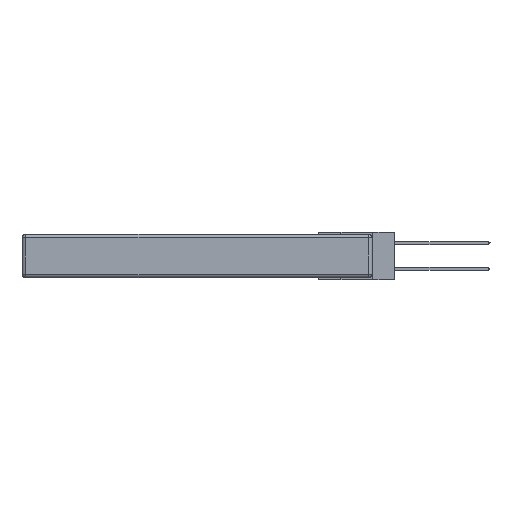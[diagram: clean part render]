
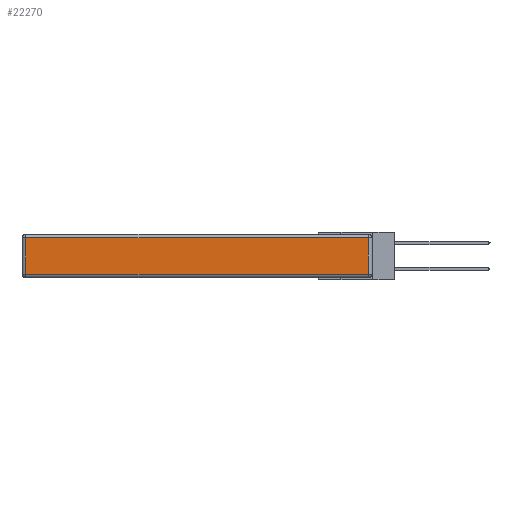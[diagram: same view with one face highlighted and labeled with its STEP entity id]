
A CAD part, left-side view. The second image highlights one B-rep face of the part: STEP entity #22270.
In plain terms, the highlighted planar face has unit normal (-1, 0, 0).
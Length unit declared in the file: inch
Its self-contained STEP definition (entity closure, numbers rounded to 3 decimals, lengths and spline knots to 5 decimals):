
#1316 = VERTEX_POINT ( 'NONE', #15758 ) ;
#3659 = CARTESIAN_POINT ( 'NONE',  ( 0., 2.72, -0.343 ) ) ;
#4221 = ORIENTED_EDGE ( 'NONE', *, *, #12453, .T. ) ;
#4222 = LINE ( 'NONE', #9980, #21115 ) ;
#4684 = CARTESIAN_POINT ( 'NONE',  ( 0., 0.03, -0.03 ) ) ;
#5134 = ORIENTED_EDGE ( 'NONE', *, *, #9528, .T. ) ;
#6177 = AXIS2_PLACEMENT_3D ( 'NONE', #9435, #19359, #13591 ) ;
#8628 = CARTESIAN_POINT ( 'NONE',  ( 0., 2.72, -0.03 ) ) ;
#9435 = CARTESIAN_POINT ( 'NONE',  ( 0., 0., -0.343 ) ) ;
#9528 = EDGE_CURVE ( 'NONE', #24288, #19897, #4222, .T. ) ;
#9539 = EDGE_CURVE ( 'NONE', #19897, #18191, #11582, .T. ) ;
#9980 = CARTESIAN_POINT ( 'NONE',  ( 0., 2.75, -0.03 ) ) ;
#10282 = VECTOR ( 'NONE', #20250, 39.37008 ) ;
#10869 = DIRECTION ( 'NONE',  ( 0., -1., 0. ) ) ;
#11462 = LINE ( 'NONE', #13032, #15913 ) ;
#11582 = LINE ( 'NONE', #3659, #10282 ) ;
#12453 = EDGE_CURVE ( 'NONE', #18191, #1316, #11462, .T. ) ;
#13032 = CARTESIAN_POINT ( 'NONE',  ( 0., 0., -0.313 ) ) ;
#13591 = DIRECTION ( 'NONE',  ( 0., 0., 1. ) ) ;
#14779 = ORIENTED_EDGE ( 'NONE', *, *, #9539, .T. ) ;
#15402 = CARTESIAN_POINT ( 'NONE',  ( 0., 2.72, -0.313 ) ) ;
#15758 = CARTESIAN_POINT ( 'NONE',  ( 0., 0.03, -0.313 ) ) ;
#15913 = VECTOR ( 'NONE', #10869, 39.37008 ) ;
#16684 = EDGE_CURVE ( 'NONE', #1316, #24288, #22419, .T. ) ;
#18191 = VERTEX_POINT ( 'NONE', #15402 ) ;
#19359 = DIRECTION ( 'NONE',  ( -1., 0., 0. ) ) ;
#19897 = VERTEX_POINT ( 'NONE', #8628 ) ;
#19948 = DIRECTION ( 'NONE',  ( 0., 0., 1. ) ) ;
#20203 = FACE_OUTER_BOUND ( 'NONE', #20688, .T. ) ;
#20250 = DIRECTION ( 'NONE',  ( 0., 0., -1. ) ) ;
#20688 = EDGE_LOOP ( 'NONE', ( #4221, #24683, #5134, #14779 ) ) ;
#21115 = VECTOR ( 'NONE', #24243, 39.37008 ) ;
#22270 = ADVANCED_FACE ( 'NONE', ( #20203 ), #25491, .T. ) ;
#22419 = LINE ( 'NONE', #23953, #24343 ) ;
#23953 = CARTESIAN_POINT ( 'NONE',  ( 0., 0.03, -0.343 ) ) ;
#24243 = DIRECTION ( 'NONE',  ( 0., 1., 0. ) ) ;
#24288 = VERTEX_POINT ( 'NONE', #4684 ) ;
#24343 = VECTOR ( 'NONE', #19948, 39.37008 ) ;
#24683 = ORIENTED_EDGE ( 'NONE', *, *, #16684, .T. ) ;
#25491 = PLANE ( 'NONE',  #6177 ) ;
